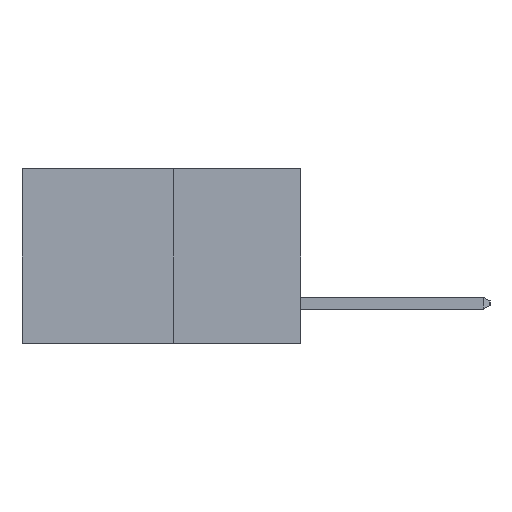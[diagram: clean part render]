
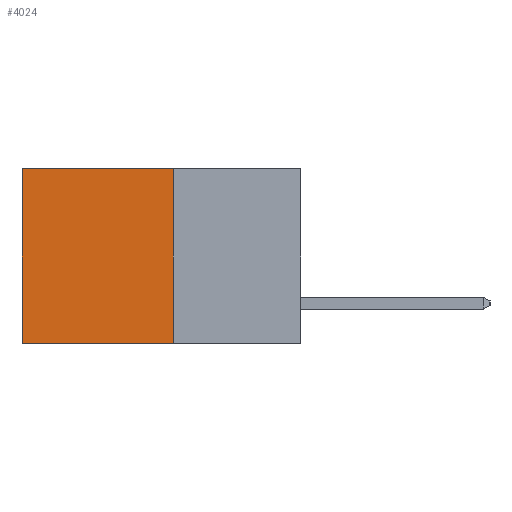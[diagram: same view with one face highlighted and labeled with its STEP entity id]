
A CAD part, left-side view. The second image highlights one B-rep face of the part: STEP entity #4024.
In plain terms, the highlighted planar face has unit normal (-1, 0, 0).
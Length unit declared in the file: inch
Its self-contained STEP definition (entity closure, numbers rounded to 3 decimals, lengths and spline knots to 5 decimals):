
#176 = AXIS2_PLACEMENT_3D ( 'NONE', #4307, #4386, #4120 ) ;
#350 = CARTESIAN_POINT ( 'NONE',  ( 0.277, 0.59, 0. ) ) ;
#544 = VERTEX_POINT ( 'NONE', #350 ) ;
#762 = LINE ( 'NONE', #8114, #8355 ) ;
#1086 = ORIENTED_EDGE ( 'NONE', *, *, #4749, .F. ) ;
#1136 = VERTEX_POINT ( 'NONE', #5954 ) ;
#1378 = EDGE_CURVE ( 'NONE', #5421, #7537, #9165, .T. ) ;
#1580 = PLANE ( 'NONE',  #176 ) ;
#2010 = EDGE_CURVE ( 'NONE', #5421, #544, #4150, .T. ) ;
#2138 = ORIENTED_EDGE ( 'NONE', *, *, #9566, .T. ) ;
#2489 = ORIENTED_EDGE ( 'NONE', *, *, #2010, .T. ) ;
#2526 = ORIENTED_EDGE ( 'NONE', *, *, #1378, .F. ) ;
#2867 = LINE ( 'NONE', #8919, #8487 ) ;
#3313 = CARTESIAN_POINT ( 'NONE',  ( 0.277, 0.27, 0. ) ) ;
#3915 = VECTOR ( 'NONE', #9528, 39.37008 ) ;
#4024 = ADVANCED_FACE ( 'NONE', ( #8701 ), #1580, .F. ) ;
#4120 = DIRECTION ( 'NONE',  ( 0., 0., -1. ) ) ;
#4150 = LINE ( 'NONE', #9619, #3915 ) ;
#4307 = CARTESIAN_POINT ( 'NONE',  ( 0.277, 0.27, -0.37 ) ) ;
#4386 = DIRECTION ( 'NONE',  ( 1., 0., 0. ) ) ;
#4749 = EDGE_CURVE ( 'NONE', #7537, #1136, #762, .T. ) ;
#4860 = CARTESIAN_POINT ( 'NONE',  ( 0.277, 0.27, -0.37 ) ) ;
#4991 = CARTESIAN_POINT ( 'NONE',  ( 0.277, 0.27, -0.37 ) ) ;
#5421 = VERTEX_POINT ( 'NONE', #3313 ) ;
#5954 = CARTESIAN_POINT ( 'NONE',  ( 0.277, 0.59, -0.37 ) ) ;
#6814 = DIRECTION ( 'NONE',  ( 0., 0., -1. ) ) ;
#7294 = DIRECTION ( 'NONE',  ( 0., 0., -1. ) ) ;
#7537 = VERTEX_POINT ( 'NONE', #4860 ) ;
#7548 = EDGE_LOOP ( 'NONE', ( #2138, #1086, #2526, #2489 ) ) ;
#8114 = CARTESIAN_POINT ( 'NONE',  ( 0.277, 0.27, -0.37 ) ) ;
#8244 = DIRECTION ( 'NONE',  ( 0., 1., 0. ) ) ;
#8355 = VECTOR ( 'NONE', #8244, 39.37008 ) ;
#8487 = VECTOR ( 'NONE', #6814, 39.37008 ) ;
#8701 = FACE_OUTER_BOUND ( 'NONE', #7548, .T. ) ;
#8919 = CARTESIAN_POINT ( 'NONE',  ( 0.277, 0.59, -0.37 ) ) ;
#8944 = VECTOR ( 'NONE', #7294, 39.37008 ) ;
#9165 = LINE ( 'NONE', #4991, #8944 ) ;
#9528 = DIRECTION ( 'NONE',  ( 0., 1., 0. ) ) ;
#9566 = EDGE_CURVE ( 'NONE', #544, #1136, #2867, .T. ) ;
#9619 = CARTESIAN_POINT ( 'NONE',  ( 0.277, 0.27, 0. ) ) ;
